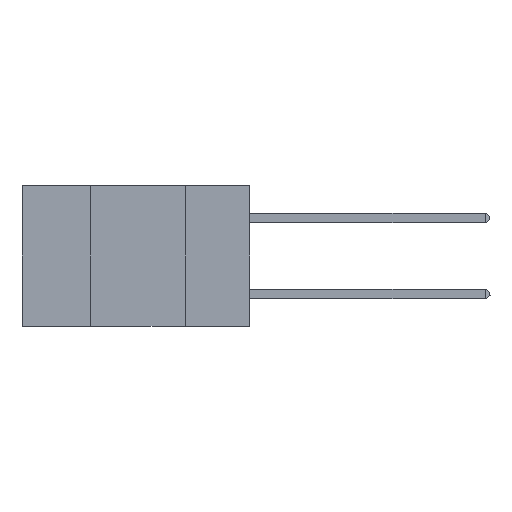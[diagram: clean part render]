
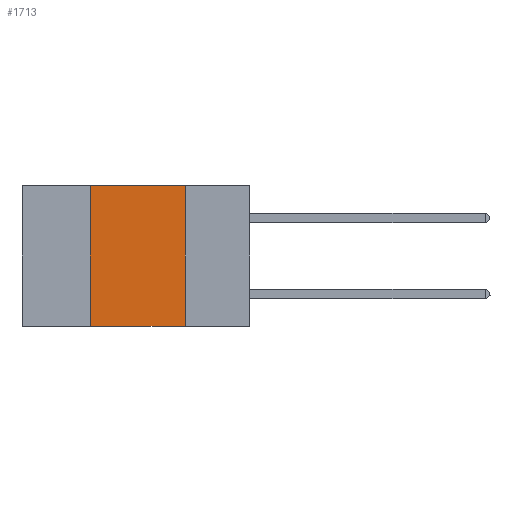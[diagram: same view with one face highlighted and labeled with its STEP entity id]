
A CAD part, left-side view. The second image highlights one B-rep face of the part: STEP entity #1713.
In plain terms, the highlighted planar face has unit normal (-1, 0, 0).
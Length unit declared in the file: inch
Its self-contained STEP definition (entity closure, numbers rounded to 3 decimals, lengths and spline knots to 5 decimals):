
#217 = CARTESIAN_POINT ( 'NONE',  ( 0., 0.42, 0. ) ) ;
#321 = CARTESIAN_POINT ( 'NONE',  ( 0., 0.17, 0. ) ) ;
#508 = EDGE_LOOP ( 'NONE', ( #3608, #5969, #1706, #12138 ) ) ;
#614 = VECTOR ( 'NONE', #756, 39.37008 ) ;
#693 = AXIS2_PLACEMENT_3D ( 'NONE', #9556, #11548, #12554 ) ;
#756 = DIRECTION ( 'NONE',  ( 0., 0., -1. ) ) ;
#844 = FACE_OUTER_BOUND ( 'NONE', #508, .T. ) ;
#1055 = CARTESIAN_POINT ( 'NONE',  ( 0., 0.17, -0.37 ) ) ;
#1229 = VERTEX_POINT ( 'NONE', #321 ) ;
#1473 = VERTEX_POINT ( 'NONE', #217 ) ;
#1706 = ORIENTED_EDGE ( 'NONE', *, *, #3526, .F. ) ;
#1713 = ADVANCED_FACE ( 'NONE', ( #844 ), #6553, .F. ) ;
#1826 = VERTEX_POINT ( 'NONE', #1055 ) ;
#2950 = DIRECTION ( 'NONE',  ( 0., 0., 1. ) ) ;
#3526 = EDGE_CURVE ( 'NONE', #10032, #1473, #10391, .T. ) ;
#3608 = ORIENTED_EDGE ( 'NONE', *, *, #12365, .F. ) ;
#4055 = CARTESIAN_POINT ( 'NONE',  ( 0., 0.42, -0.37 ) ) ;
#4931 = EDGE_CURVE ( 'NONE', #10032, #1826, #5675, .T. ) ;
#5546 = EDGE_CURVE ( 'NONE', #1473, #1229, #8900, .T. ) ;
#5675 = LINE ( 'NONE', #12476, #10350 ) ;
#5886 = LINE ( 'NONE', #11642, #614 ) ;
#5969 = ORIENTED_EDGE ( 'NONE', *, *, #5546, .F. ) ;
#6526 = DIRECTION ( 'NONE',  ( 0., -1., 0. ) ) ;
#6553 = PLANE ( 'NONE',  #693 ) ;
#8490 = VECTOR ( 'NONE', #2950, 39.37008 ) ;
#8900 = LINE ( 'NONE', #9072, #12339 ) ;
#9072 = CARTESIAN_POINT ( 'NONE',  ( 0., 0.6, 0. ) ) ;
#9556 = CARTESIAN_POINT ( 'NONE',  ( 0., 0.6, 0. ) ) ;
#10032 = VERTEX_POINT ( 'NONE', #4055 ) ;
#10350 = VECTOR ( 'NONE', #6526, 39.37008 ) ;
#10391 = LINE ( 'NONE', #12851, #8490 ) ;
#11548 = DIRECTION ( 'NONE',  ( 1., 0., 0. ) ) ;
#11642 = CARTESIAN_POINT ( 'NONE',  ( 0., 0.17, 0. ) ) ;
#11945 = DIRECTION ( 'NONE',  ( 0., -1., 0. ) ) ;
#12138 = ORIENTED_EDGE ( 'NONE', *, *, #4931, .T. ) ;
#12339 = VECTOR ( 'NONE', #11945, 39.37008 ) ;
#12365 = EDGE_CURVE ( 'NONE', #1229, #1826, #5886, .T. ) ;
#12476 = CARTESIAN_POINT ( 'NONE',  ( 0., 0.6, -0.37 ) ) ;
#12554 = DIRECTION ( 'NONE',  ( 0., 0., -1. ) ) ;
#12851 = CARTESIAN_POINT ( 'NONE',  ( 0., 0.42, 0. ) ) ;
